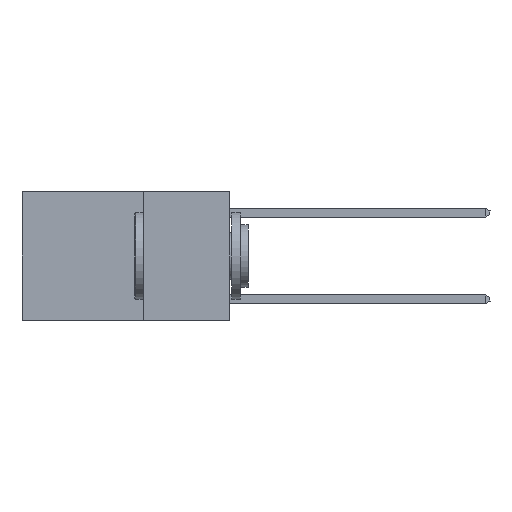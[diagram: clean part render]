
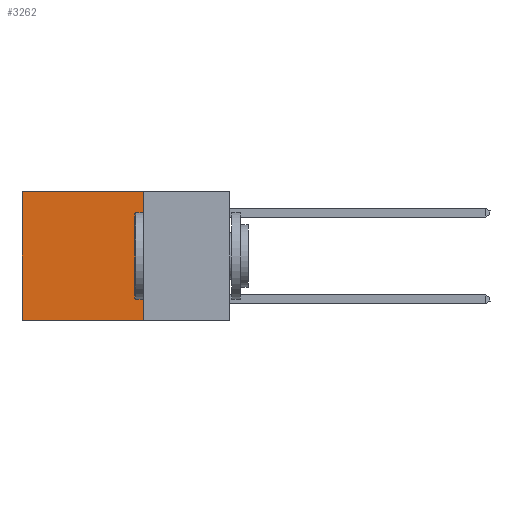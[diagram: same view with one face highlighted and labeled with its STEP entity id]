
A CAD part, left-side view. The second image highlights one B-rep face of the part: STEP entity #3262.
In plain terms, the highlighted planar face has unit normal (-1, 0, 0).
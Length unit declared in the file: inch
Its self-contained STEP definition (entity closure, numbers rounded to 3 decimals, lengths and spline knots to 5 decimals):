
#69 = DIRECTION ( 'NONE',  ( 0., 0., -1. ) ) ;
#177 = ORIENTED_EDGE ( 'NONE', *, *, #10186, .F. ) ;
#281 = VERTEX_POINT ( 'NONE', #2796 ) ;
#803 = EDGE_CURVE ( 'NONE', #12001, #10324, #2428, .T. ) ;
#1033 = DIRECTION ( 'NONE',  ( 1., 0., 0. ) ) ;
#1414 = CARTESIAN_POINT ( 'NONE',  ( 0.2625, 0.6, 0. ) ) ;
#1607 = CARTESIAN_POINT ( 'NONE',  ( 0.2625, 0.25, 0. ) ) ;
#2299 = CARTESIAN_POINT ( 'NONE',  ( 0.2625, 0.25, -0.37 ) ) ;
#2428 = LINE ( 'NONE', #7449, #5956 ) ;
#2542 = DIRECTION ( 'NONE',  ( 0., 0., -1. ) ) ;
#2673 = EDGE_LOOP ( 'NONE', ( #7741, #11917, #177, #5383 ) ) ;
#2796 = CARTESIAN_POINT ( 'NONE',  ( 0.2625, 0.6, -0.37 ) ) ;
#2943 = FACE_OUTER_BOUND ( 'NONE', #2673, .T. ) ;
#2946 = CARTESIAN_POINT ( 'NONE',  ( 0.2625, 0.6, 0. ) ) ;
#2980 = LINE ( 'NONE', #2299, #4955 ) ;
#3262 = ADVANCED_FACE ( 'NONE', ( #2943 ), #10603, .F. ) ;
#3395 = DIRECTION ( 'NONE',  ( 0., 1., 0. ) ) ;
#3587 = AXIS2_PLACEMENT_3D ( 'NONE', #5846, #1033, #69 ) ;
#4270 = CARTESIAN_POINT ( 'NONE',  ( 0.2625, 0.25, -0.37 ) ) ;
#4450 = LINE ( 'NONE', #1414, #5916 ) ;
#4955 = VECTOR ( 'NONE', #11454, 39.37008 ) ;
#5171 = CARTESIAN_POINT ( 'NONE',  ( 0.2625, 0.25, 0. ) ) ;
#5246 = DIRECTION ( 'NONE',  ( 0., 0., -1. ) ) ;
#5383 = ORIENTED_EDGE ( 'NONE', *, *, #803, .T. ) ;
#5439 = EDGE_CURVE ( 'NONE', #11862, #281, #2980, .T. ) ;
#5661 = LINE ( 'NONE', #1607, #8710 ) ;
#5846 = CARTESIAN_POINT ( 'NONE',  ( 0.2625, 0.25, 0. ) ) ;
#5916 = VECTOR ( 'NONE', #5246, 39.37008 ) ;
#5956 = VECTOR ( 'NONE', #3395, 39.37008 ) ;
#7449 = CARTESIAN_POINT ( 'NONE',  ( 0.2625, 0.25, 0. ) ) ;
#7741 = ORIENTED_EDGE ( 'NONE', *, *, #9118, .T. ) ;
#8710 = VECTOR ( 'NONE', #2542, 39.37008 ) ;
#9118 = EDGE_CURVE ( 'NONE', #10324, #281, #4450, .T. ) ;
#10186 = EDGE_CURVE ( 'NONE', #12001, #11862, #5661, .T. ) ;
#10324 = VERTEX_POINT ( 'NONE', #2946 ) ;
#10603 = PLANE ( 'NONE',  #3587 ) ;
#11454 = DIRECTION ( 'NONE',  ( 0., 1., 0. ) ) ;
#11862 = VERTEX_POINT ( 'NONE', #4270 ) ;
#11917 = ORIENTED_EDGE ( 'NONE', *, *, #5439, .F. ) ;
#12001 = VERTEX_POINT ( 'NONE', #5171 ) ;
